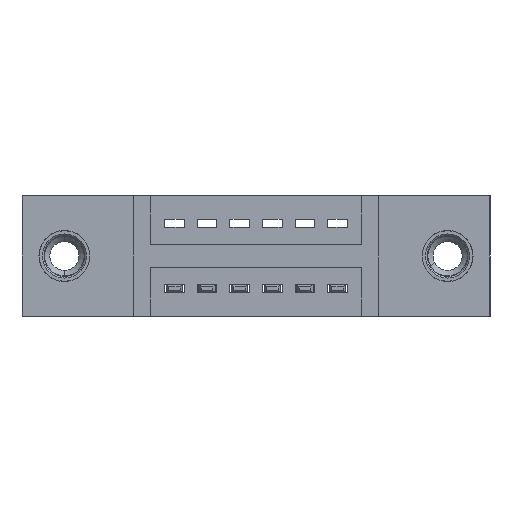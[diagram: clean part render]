
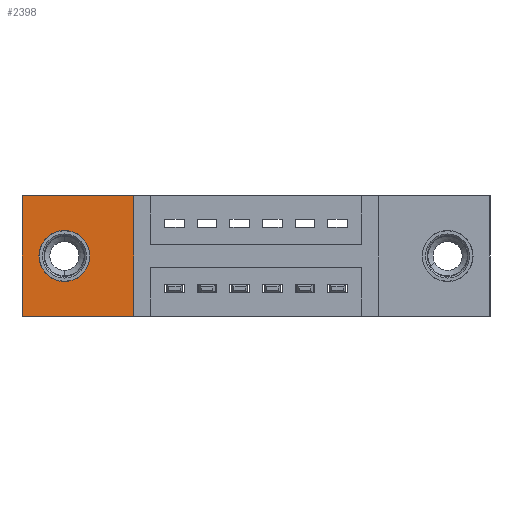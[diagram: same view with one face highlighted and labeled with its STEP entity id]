
A CAD part, front view. The second image highlights one B-rep face of the part: STEP entity #2398.
In plain terms, the highlighted planar face has unit normal (0, -1, 0).
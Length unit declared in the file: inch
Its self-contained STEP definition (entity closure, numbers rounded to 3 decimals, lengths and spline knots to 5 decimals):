
#141 = ORIENTED_EDGE ( 'NONE', *, *, #9099, .F. ) ;
#210 = AXIS2_PLACEMENT_3D ( 'NONE', #630, #3783, #2885 ) ;
#630 = CARTESIAN_POINT ( 'NONE',  ( 0., 0.11, -0.37 ) ) ;
#642 = AXIS2_PLACEMENT_3D ( 'NONE', #3507, #8468, #10102 ) ;
#666 = VERTEX_POINT ( 'NONE', #4431 ) ;
#721 = DIRECTION ( 'NONE',  ( -1., 0., 0. ) ) ;
#1645 = VECTOR ( 'NONE', #3918, 39.37008 ) ;
#1992 = VERTEX_POINT ( 'NONE', #5624 ) ;
#2089 = CARTESIAN_POINT ( 'NONE',  ( 0.3425, 0.11, 0. ) ) ;
#2398 = ADVANCED_FACE ( 'NONE', ( #9085, #5263 ), #9599, .T. ) ;
#2568 = AXIS2_PLACEMENT_3D ( 'NONE', #9214, #3502, #6810 ) ;
#2885 = DIRECTION ( 'NONE',  ( 0., 0., -1. ) ) ;
#2894 = ORIENTED_EDGE ( 'NONE', *, *, #8134, .T. ) ;
#2906 = DIRECTION ( 'NONE',  ( 0., 0., 1. ) ) ;
#3502 = DIRECTION ( 'NONE',  ( 0., -1., 0. ) ) ;
#3507 = CARTESIAN_POINT ( 'NONE',  ( 0.13, 0.11, -0.185 ) ) ;
#3783 = DIRECTION ( 'NONE',  ( 0., -1., 0. ) ) ;
#3918 = DIRECTION ( 'NONE',  ( 0., 0., -1. ) ) ;
#3943 = CARTESIAN_POINT ( 'NONE',  ( 0., 0.11, -0.37 ) ) ;
#4431 = CARTESIAN_POINT ( 'NONE',  ( 0.13, 0.11, -0.263 ) ) ;
#4494 = ORIENTED_EDGE ( 'NONE', *, *, #10182, .F. ) ;
#4543 = VECTOR ( 'NONE', #2906, 39.37008 ) ;
#4915 = VERTEX_POINT ( 'NONE', #9311 ) ;
#5059 = CARTESIAN_POINT ( 'NONE',  ( 0.3425, 0.11, -0.37 ) ) ;
#5195 = LINE ( 'NONE', #3943, #9496 ) ;
#5263 = FACE_OUTER_BOUND ( 'NONE', #5601, .T. ) ;
#5601 = EDGE_LOOP ( 'NONE', ( #5846, #10383, #2894, #6198 ) ) ;
#5624 = CARTESIAN_POINT ( 'NONE',  ( 0.3425, 0.11, 0. ) ) ;
#5846 = ORIENTED_EDGE ( 'NONE', *, *, #6014, .T. ) ;
#6014 = EDGE_CURVE ( 'NONE', #8889, #4915, #7470, .T. ) ;
#6039 = CARTESIAN_POINT ( 'NONE',  ( 0., 0.11, 0. ) ) ;
#6198 = ORIENTED_EDGE ( 'NONE', *, *, #6692, .T. ) ;
#6692 = EDGE_CURVE ( 'NONE', #1992, #8889, #10169, .T. ) ;
#6810 = DIRECTION ( 'NONE',  ( 0., 0., -1. ) ) ;
#7079 = CARTESIAN_POINT ( 'NONE',  ( 0.13, 0.11, -0.107 ) ) ;
#7296 = CIRCLE ( 'NONE', #642, 0.078 ) ;
#7470 = LINE ( 'NONE', #10309, #1645 ) ;
#8134 = EDGE_CURVE ( 'NONE', #10196, #1992, #9913, .T. ) ;
#8468 = DIRECTION ( 'NONE',  ( 0., -1., 0. ) ) ;
#8721 = CIRCLE ( 'NONE', #2568, 0.078 ) ;
#8773 = EDGE_CURVE ( 'NONE', #4915, #10196, #5195, .T. ) ;
#8889 = VERTEX_POINT ( 'NONE', #6039 ) ;
#8915 = CARTESIAN_POINT ( 'NONE',  ( 0., 0.11, 0. ) ) ;
#9085 = FACE_BOUND ( 'NONE', #10232, .T. ) ;
#9099 = EDGE_CURVE ( 'NONE', #666, #9220, #8721, .T. ) ;
#9214 = CARTESIAN_POINT ( 'NONE',  ( 0.13, 0.11, -0.185 ) ) ;
#9220 = VERTEX_POINT ( 'NONE', #7079 ) ;
#9311 = CARTESIAN_POINT ( 'NONE',  ( 0., 0.11, -0.37 ) ) ;
#9496 = VECTOR ( 'NONE', #10438, 39.37008 ) ;
#9599 = PLANE ( 'NONE',  #210 ) ;
#9607 = VECTOR ( 'NONE', #721, 39.37008 ) ;
#9913 = LINE ( 'NONE', #2089, #4543 ) ;
#10102 = DIRECTION ( 'NONE',  ( 0., 0., -1. ) ) ;
#10169 = LINE ( 'NONE', #8915, #9607 ) ;
#10182 = EDGE_CURVE ( 'NONE', #9220, #666, #7296, .T. ) ;
#10196 = VERTEX_POINT ( 'NONE', #5059 ) ;
#10232 = EDGE_LOOP ( 'NONE', ( #4494, #141 ) ) ;
#10309 = CARTESIAN_POINT ( 'NONE',  ( 0., 0.11, 0. ) ) ;
#10383 = ORIENTED_EDGE ( 'NONE', *, *, #8773, .T. ) ;
#10438 = DIRECTION ( 'NONE',  ( 1., 0., 0. ) ) ;
